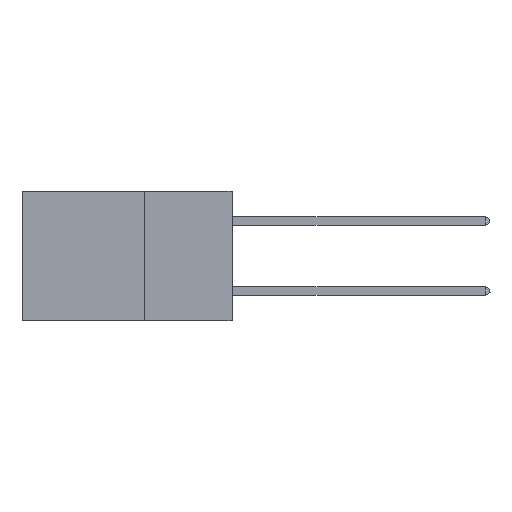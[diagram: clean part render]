
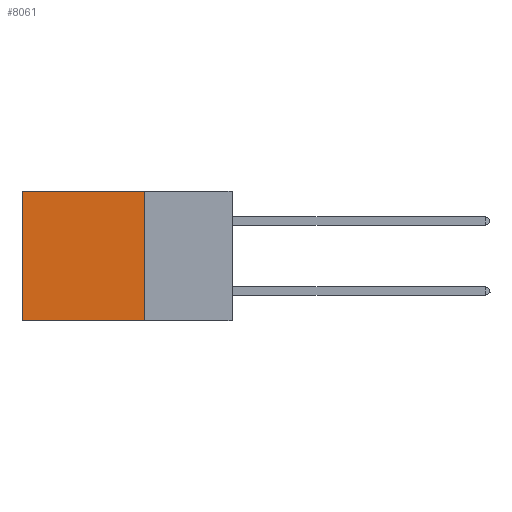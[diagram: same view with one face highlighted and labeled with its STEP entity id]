
A CAD part, left-side view. The second image highlights one B-rep face of the part: STEP entity #8061.
In plain terms, the highlighted planar face has unit normal (-1, 0, 0).
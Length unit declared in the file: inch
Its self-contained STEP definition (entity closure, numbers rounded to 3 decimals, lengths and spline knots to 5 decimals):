
#226 = FACE_OUTER_BOUND ( 'NONE', #14416, .T. ) ;
#521 = CARTESIAN_POINT ( 'NONE',  ( 0.2875, 0.25, -0.37 ) ) ;
#568 = LINE ( 'NONE', #1581, #10017 ) ;
#579 = DIRECTION ( 'NONE',  ( 0., 0., -1. ) ) ;
#971 = DIRECTION ( 'NONE',  ( 0., 1., 0. ) ) ;
#1068 = DIRECTION ( 'NONE',  ( 0., 1., 0. ) ) ;
#1581 = CARTESIAN_POINT ( 'NONE',  ( 0.2875, 0.25, 0. ) ) ;
#1594 = LINE ( 'NONE', #521, #11869 ) ;
#1771 = CARTESIAN_POINT ( 'NONE',  ( 0.2875, 0.6, 0. ) ) ;
#2453 = CARTESIAN_POINT ( 'NONE',  ( 0.2875, 0.6, 0. ) ) ;
#3108 = VECTOR ( 'NONE', #3895, 39.37008 ) ;
#3236 = CARTESIAN_POINT ( 'NONE',  ( 0.2875, 0.25, 0. ) ) ;
#3405 = VERTEX_POINT ( 'NONE', #10631 ) ;
#3895 = DIRECTION ( 'NONE',  ( 0., 0., -1. ) ) ;
#4075 = LINE ( 'NONE', #15827, #7434 ) ;
#4154 = AXIS2_PLACEMENT_3D ( 'NONE', #3236, #16777, #579 ) ;
#5443 = EDGE_CURVE ( 'NONE', #16803, #6421, #568, .T. ) ;
#5585 = ORIENTED_EDGE ( 'NONE', *, *, #6000, .F. ) ;
#6000 = EDGE_CURVE ( 'NONE', #6421, #3405, #1594, .T. ) ;
#6421 = VERTEX_POINT ( 'NONE', #14389 ) ;
#6834 = LINE ( 'NONE', #2453, #3108 ) ;
#6885 = EDGE_CURVE ( 'NONE', #16803, #10066, #4075, .T. ) ;
#7434 = VECTOR ( 'NONE', #1068, 39.37008 ) ;
#8061 = ADVANCED_FACE ( 'NONE', ( #226 ), #8558, .F. ) ;
#8558 = PLANE ( 'NONE',  #4154 ) ;
#10017 = VECTOR ( 'NONE', #14889, 39.37008 ) ;
#10066 = VERTEX_POINT ( 'NONE', #1771 ) ;
#10631 = CARTESIAN_POINT ( 'NONE',  ( 0.2875, 0.6, -0.37 ) ) ;
#11631 = ORIENTED_EDGE ( 'NONE', *, *, #5443, .F. ) ;
#11869 = VECTOR ( 'NONE', #971, 39.37008 ) ;
#12202 = ORIENTED_EDGE ( 'NONE', *, *, #6885, .T. ) ;
#12763 = CARTESIAN_POINT ( 'NONE',  ( 0.2875, 0.25, 0. ) ) ;
#13034 = EDGE_CURVE ( 'NONE', #10066, #3405, #6834, .T. ) ;
#14389 = CARTESIAN_POINT ( 'NONE',  ( 0.2875, 0.25, -0.37 ) ) ;
#14416 = EDGE_LOOP ( 'NONE', ( #14693, #5585, #11631, #12202 ) ) ;
#14693 = ORIENTED_EDGE ( 'NONE', *, *, #13034, .T. ) ;
#14889 = DIRECTION ( 'NONE',  ( 0., 0., -1. ) ) ;
#15827 = CARTESIAN_POINT ( 'NONE',  ( 0.2875, 0.25, 0. ) ) ;
#16777 = DIRECTION ( 'NONE',  ( 1., 0., 0. ) ) ;
#16803 = VERTEX_POINT ( 'NONE', #12763 ) ;
